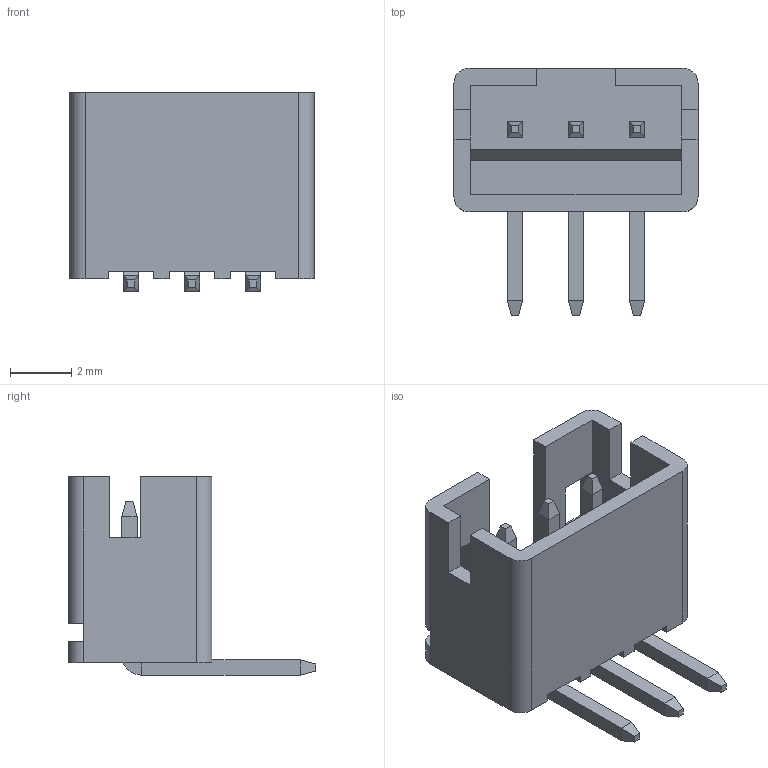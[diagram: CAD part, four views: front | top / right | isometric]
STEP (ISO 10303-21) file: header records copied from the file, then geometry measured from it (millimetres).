
FILE_DESCRIPTION (( 'STEP AP203' ), '1' );
FILE_NAME ('140-503-415-100.STEP', '2020-09-25T10:59:01', ( '' ), ( '' ), 'SwSTEP 2.0', 'SolidWorks 2020', '' );
FILE_SCHEMA (( 'CONFIG_CONTROL_DESIGN' ));
Length unit declared in the file: millimetre
Products named in the file (3): RA LI Contact_Str; 140-503-415-100; RA LI Housing_503
Assembly tree (4 placements, depth 2):
  140-503-415-100
    RA LI Housing_503
    RA LI Contact_Str  x3
Bounding box: 8 x 8.1 x 6.5 mm (x, y, z)
Volume: 102.4 mm3; surface area: 387.2 mm2
Topology: 4 solids, 4 shells, 130 faces, 320 edges, 196 vertices
Faces by surface type: plane 118, cylinder 12
Entity records: 3021 total; most frequent: CARTESIAN_POINT 473, ORIENTED_EDGE 464, DIRECTION 434, EDGE_CURVE 232, LINE 216, VECTOR 216, VERTEX_POINT 148, AXIS2_PLACEMENT_3D 109
